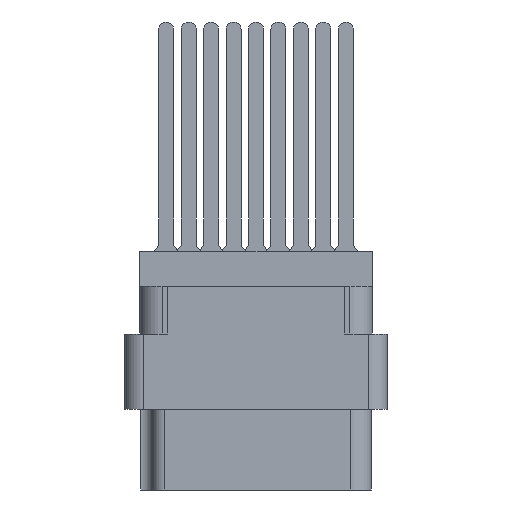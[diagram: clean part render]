
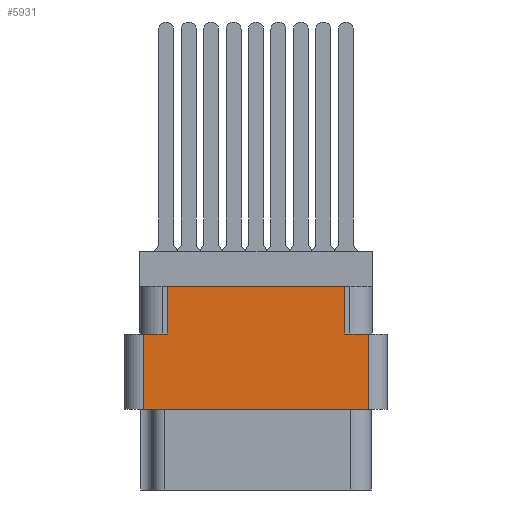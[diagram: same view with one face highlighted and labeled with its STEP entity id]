
A CAD part, left-side view. The second image highlights one B-rep face of the part: STEP entity #5931.
In plain terms, the highlighted planar face has unit normal (-1, 0, 0).
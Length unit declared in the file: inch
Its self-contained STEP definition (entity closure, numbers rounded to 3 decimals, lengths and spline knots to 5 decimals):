
#352 = CARTESIAN_POINT ( 'NONE',  ( -1.296, -0.438, -0.798 ) ) ;
#430 = EDGE_CURVE ( 'NONE', #32108, #21439, #40984, .T. ) ;
#744 = CARTESIAN_POINT ( 'NONE',  ( -1.296, -0.296, -0.117 ) ) ;
#1212 = VERTEX_POINT ( 'NONE', #9117 ) ;
#1998 = CARTESIAN_POINT ( 'NONE',  ( -1.296, -0.376, -0.277 ) ) ;
#3351 = EDGE_CURVE ( 'NONE', #24458, #45759, #45745, .T. ) ;
#4184 = EDGE_LOOP ( 'NONE', ( #34219, #40985, #31340, #20012, #41470, #29742, #39755, #31639 ) ) ;
#5120 = CARTESIAN_POINT ( 'NONE',  ( -1.296, 0., -0.277 ) ) ;
#5187 = VECTOR ( 'NONE', #41565, 39.37008 ) ;
#5244 = EDGE_CURVE ( 'NONE', #33966, #40505, #24006, .T. ) ;
#5931 = ADVANCED_FACE ( 'NONE', ( #26167 ), #44100, .T. ) ;
#7388 = CARTESIAN_POINT ( 'NONE',  ( -1.296, 0.376, -0.277 ) ) ;
#8099 = EDGE_CURVE ( 'NONE', #45759, #21439, #43160, .T. ) ;
#9117 = CARTESIAN_POINT ( 'NONE',  ( -1.296, -0.376, -0.529 ) ) ;
#10128 = DIRECTION ( 'NONE',  ( 0., 0., 1. ) ) ;
#10537 = CARTESIAN_POINT ( 'NONE',  ( -1.296, 0.296, -0.277 ) ) ;
#11213 = CARTESIAN_POINT ( 'NONE',  ( -1.296, 0.376, -0.798 ) ) ;
#11396 = CARTESIAN_POINT ( 'NONE',  ( -1.296, 0.376, -0.529 ) ) ;
#11555 = CARTESIAN_POINT ( 'NONE',  ( -1.296, -0.296, -0.277 ) ) ;
#13010 = CARTESIAN_POINT ( 'NONE',  ( -1.296, 0.296, -0.117 ) ) ;
#15477 = VECTOR ( 'NONE', #31172, 39.37008 ) ;
#18739 = VERTEX_POINT ( 'NONE', #1998 ) ;
#18856 = DIRECTION ( 'NONE',  ( 0., 0., 1. ) ) ;
#19633 = VECTOR ( 'NONE', #24898, 39.37008 ) ;
#19760 = AXIS2_PLACEMENT_3D ( 'NONE', #352, #40183, #18856 ) ;
#20012 = ORIENTED_EDGE ( 'NONE', *, *, #22523, .T. ) ;
#21439 = VERTEX_POINT ( 'NONE', #744 ) ;
#22523 = EDGE_CURVE ( 'NONE', #1212, #18739, #24558, .T. ) ;
#24006 = LINE ( 'NONE', #11213, #46753 ) ;
#24458 = VERTEX_POINT ( 'NONE', #10537 ) ;
#24558 = LINE ( 'NONE', #38051, #5187 ) ;
#24898 = DIRECTION ( 'NONE',  ( 0., 1., 0. ) ) ;
#25863 = DIRECTION ( 'NONE',  ( 0., 0., -1. ) ) ;
#25901 = DIRECTION ( 'NONE',  ( 0., 0., 1. ) ) ;
#26167 = FACE_OUTER_BOUND ( 'NONE', #4184, .T. ) ;
#26384 = VECTOR ( 'NONE', #10128, 39.37008 ) ;
#29246 = LINE ( 'NONE', #42892, #19633 ) ;
#29742 = ORIENTED_EDGE ( 'NONE', *, *, #430, .T. ) ;
#30472 = EDGE_CURVE ( 'NONE', #1212, #40505, #29246, .T. ) ;
#30710 = DIRECTION ( 'NONE',  ( 0., -1., 0. ) ) ;
#31172 = DIRECTION ( 'NONE',  ( 0., -1., 0. ) ) ;
#31340 = ORIENTED_EDGE ( 'NONE', *, *, #30472, .F. ) ;
#31639 = ORIENTED_EDGE ( 'NONE', *, *, #3351, .F. ) ;
#31921 = CARTESIAN_POINT ( 'NONE',  ( -1.296, 0.296, -0.277 ) ) ;
#32108 = VERTEX_POINT ( 'NONE', #41185 ) ;
#32629 = CARTESIAN_POINT ( 'NONE',  ( -1.296, 0.438, -0.117 ) ) ;
#33497 = VECTOR ( 'NONE', #30710, 39.37008 ) ;
#33507 = VECTOR ( 'NONE', #36453, 39.37008 ) ;
#33966 = VERTEX_POINT ( 'NONE', #7388 ) ;
#34175 = EDGE_CURVE ( 'NONE', #33966, #24458, #36893, .T. ) ;
#34219 = ORIENTED_EDGE ( 'NONE', *, *, #34175, .F. ) ;
#34723 = CARTESIAN_POINT ( 'NONE',  ( -1.296, 0., -0.277 ) ) ;
#36453 = DIRECTION ( 'NONE',  ( 0., -1., 0. ) ) ;
#36893 = LINE ( 'NONE', #5120, #33497 ) ;
#37522 = VECTOR ( 'NONE', #25901, 39.37008 ) ;
#38051 = CARTESIAN_POINT ( 'NONE',  ( -1.296, -0.376, -0.798 ) ) ;
#38142 = EDGE_CURVE ( 'NONE', #32108, #18739, #43892, .T. ) ;
#39755 = ORIENTED_EDGE ( 'NONE', *, *, #8099, .F. ) ;
#40183 = DIRECTION ( 'NONE',  ( -1., 0., 0. ) ) ;
#40505 = VERTEX_POINT ( 'NONE', #11396 ) ;
#40984 = LINE ( 'NONE', #11555, #37522 ) ;
#40985 = ORIENTED_EDGE ( 'NONE', *, *, #5244, .T. ) ;
#41185 = CARTESIAN_POINT ( 'NONE',  ( -1.296, -0.296, -0.277 ) ) ;
#41470 = ORIENTED_EDGE ( 'NONE', *, *, #38142, .F. ) ;
#41565 = DIRECTION ( 'NONE',  ( 0., 0., 1. ) ) ;
#42892 = CARTESIAN_POINT ( 'NONE',  ( -1.296, 0., -0.529 ) ) ;
#43160 = LINE ( 'NONE', #32629, #33507 ) ;
#43892 = LINE ( 'NONE', #34723, #15477 ) ;
#44100 = PLANE ( 'NONE',  #19760 ) ;
#45745 = LINE ( 'NONE', #31921, #26384 ) ;
#45759 = VERTEX_POINT ( 'NONE', #13010 ) ;
#46753 = VECTOR ( 'NONE', #25863, 39.37008 ) ;
